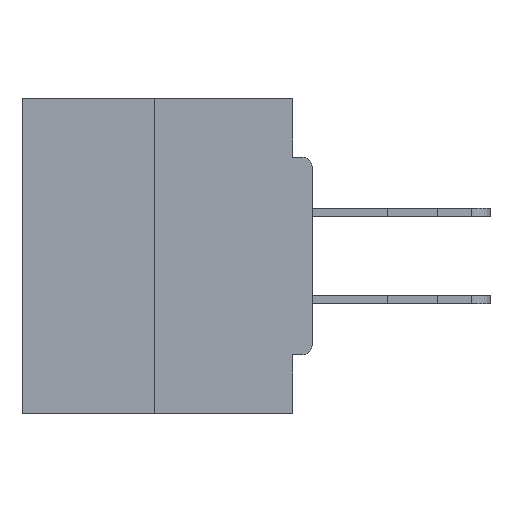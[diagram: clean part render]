
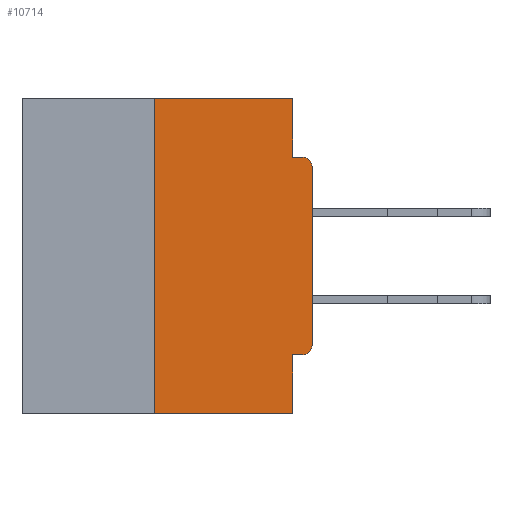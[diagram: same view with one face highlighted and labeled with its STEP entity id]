
A CAD part, left-side view. The second image highlights one B-rep face of the part: STEP entity #10714.
In plain terms, the highlighted planar face has unit normal (-1, 0, 0).
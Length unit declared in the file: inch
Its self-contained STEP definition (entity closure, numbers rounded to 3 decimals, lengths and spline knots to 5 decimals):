
#141 = ORIENTED_EDGE ( 'NONE', *, *, #17769, .T. ) ;
#172 = DIRECTION ( 'NONE',  ( 0., 0., -1. ) ) ;
#173 = DIRECTION ( 'NONE',  ( 0., -1., 0. ) ) ;
#638 = LINE ( 'NONE', #19445, #23452 ) ;
#1188 = CARTESIAN_POINT ( 'NONE',  ( 0., 0., 0. ) ) ;
#2145 = CARTESIAN_POINT ( 'NONE',  ( 0., 0.25, 0. ) ) ;
#2170 = LINE ( 'NONE', #11632, #36227 ) ;
#2729 = DIRECTION ( 'NONE',  ( 0., -1., 0. ) ) ;
#3438 = CARTESIAN_POINT ( 'NONE',  ( 0., 0.015, -0.3915 ) ) ;
#3566 = DIRECTION ( 'NONE',  ( 0., 0., 1. ) ) ;
#4624 = EDGE_CURVE ( 'NONE', #17045, #29672, #16320, .T. ) ;
#4887 = CARTESIAN_POINT ( 'NONE',  ( 0., 0.015, -0.0935 ) ) ;
#5136 = EDGE_CURVE ( 'NONE', #35046, #29506, #31092, .T. ) ;
#5449 = EDGE_CURVE ( 'NONE', #21550, #13218, #638, .T. ) ;
#6110 = AXIS2_PLACEMENT_3D ( 'NONE', #3438, #6583, #9461 ) ;
#6583 = DIRECTION ( 'NONE',  ( -1., 0., 0. ) ) ;
#6952 = CARTESIAN_POINT ( 'NONE',  ( 0., 0.031, -0.5 ) ) ;
#7088 = ORIENTED_EDGE ( 'NONE', *, *, #30338, .T. ) ;
#7801 = DIRECTION ( 'NONE',  ( 0., -1., 0. ) ) ;
#8574 = CIRCLE ( 'NONE', #6110, 0.015 ) ;
#8868 = CARTESIAN_POINT ( 'NONE',  ( 0., 0., -0.4065 ) ) ;
#9128 = CARTESIAN_POINT ( 'NONE',  ( 0., 0.031, -0.4065 ) ) ;
#9140 = EDGE_LOOP ( 'NONE', ( #13196, #24251, #141, #27956, #31343, #7088, #16953, #16206, #29349, #14615 ) ) ;
#9144 = CARTESIAN_POINT ( 'NONE',  ( 0., 0.46, 0. ) ) ;
#9461 = DIRECTION ( 'NONE',  ( 0., 0., -1. ) ) ;
#9578 = CARTESIAN_POINT ( 'NONE',  ( 0., 0.25, -0.5 ) ) ;
#9580 = DIRECTION ( 'NONE',  ( 0., 0., -1. ) ) ;
#9927 = EDGE_CURVE ( 'NONE', #35628, #25838, #33944, .T. ) ;
#10643 = AXIS2_PLACEMENT_3D ( 'NONE', #9144, #23290, #172 ) ;
#10714 = ADVANCED_FACE ( 'NONE', ( #15776 ), #11755, .F. ) ;
#10856 = CARTESIAN_POINT ( 'NONE',  ( 0., 0., -0.3915 ) ) ;
#11632 = CARTESIAN_POINT ( 'NONE',  ( 0., 0.46, -0.5 ) ) ;
#11755 = PLANE ( 'NONE',  #10643 ) ;
#12730 = CARTESIAN_POINT ( 'NONE',  ( 0., 0.031, -0.0935 ) ) ;
#12836 = CARTESIAN_POINT ( 'NONE',  ( 0., 0.46, 0. ) ) ;
#13103 = VERTEX_POINT ( 'NONE', #29888 ) ;
#13196 = ORIENTED_EDGE ( 'NONE', *, *, #21274, .F. ) ;
#13218 = VERTEX_POINT ( 'NONE', #4887 ) ;
#13568 = CIRCLE ( 'NONE', #36245, 0.015 ) ;
#14615 = ORIENTED_EDGE ( 'NONE', *, *, #32724, .F. ) ;
#14978 = DIRECTION ( 'NONE',  ( 0., 0., -1. ) ) ;
#14980 = VECTOR ( 'NONE', #28480, 39.37008 ) ;
#15696 = EDGE_CURVE ( 'NONE', #29672, #34847, #34263, .T. ) ;
#15776 = FACE_OUTER_BOUND ( 'NONE', #9140, .T. ) ;
#16206 = ORIENTED_EDGE ( 'NONE', *, *, #28517, .T. ) ;
#16320 = LINE ( 'NONE', #8868, #14980 ) ;
#16727 = CARTESIAN_POINT ( 'NONE',  ( 0., 0.25, 0. ) ) ;
#16953 = ORIENTED_EDGE ( 'NONE', *, *, #5136, .T. ) ;
#17045 = VERTEX_POINT ( 'NONE', #33713 ) ;
#17710 = VECTOR ( 'NONE', #14978, 39.37008 ) ;
#17769 = EDGE_CURVE ( 'NONE', #35628, #34847, #2170, .T. ) ;
#18042 = DIRECTION ( 'NONE',  ( 0., 0., -1. ) ) ;
#18284 = DIRECTION ( 'NONE',  ( -1., 0., 0. ) ) ;
#19445 = CARTESIAN_POINT ( 'NONE',  ( 0., 0., -0.0935 ) ) ;
#21274 = EDGE_CURVE ( 'NONE', #25838, #13103, #27729, .T. ) ;
#21550 = VERTEX_POINT ( 'NONE', #12730 ) ;
#23290 = DIRECTION ( 'NONE',  ( 1., 0., 0. ) ) ;
#23452 = VECTOR ( 'NONE', #7801, 39.37008 ) ;
#24002 = CARTESIAN_POINT ( 'NONE',  ( 0., 0.031, -0.5 ) ) ;
#24251 = ORIENTED_EDGE ( 'NONE', *, *, #9927, .F. ) ;
#25406 = CARTESIAN_POINT ( 'NONE',  ( 0., 0., -0.1085 ) ) ;
#25838 = VERTEX_POINT ( 'NONE', #16727 ) ;
#26329 = VECTOR ( 'NONE', #30411, 39.37008 ) ;
#26729 = LINE ( 'NONE', #35127, #29843 ) ;
#27729 = LINE ( 'NONE', #12836, #36725 ) ;
#27956 = ORIENTED_EDGE ( 'NONE', *, *, #15696, .F. ) ;
#28369 = VECTOR ( 'NONE', #3566, 39.37008 ) ;
#28480 = DIRECTION ( 'NONE',  ( 0., 1., 0. ) ) ;
#28517 = EDGE_CURVE ( 'NONE', #29506, #13218, #13568, .T. ) ;
#29349 = ORIENTED_EDGE ( 'NONE', *, *, #5449, .F. ) ;
#29506 = VERTEX_POINT ( 'NONE', #25406 ) ;
#29672 = VERTEX_POINT ( 'NONE', #9128 ) ;
#29843 = VECTOR ( 'NONE', #9580, 39.37008 ) ;
#29888 = CARTESIAN_POINT ( 'NONE',  ( 0., 0.031, 0. ) ) ;
#30338 = EDGE_CURVE ( 'NONE', #17045, #35046, #8574, .T. ) ;
#30411 = DIRECTION ( 'NONE',  ( 0., 0., 1. ) ) ;
#31092 = LINE ( 'NONE', #1188, #28369 ) ;
#31343 = ORIENTED_EDGE ( 'NONE', *, *, #4624, .F. ) ;
#32666 = CARTESIAN_POINT ( 'NONE',  ( 0., 0.015, -0.1085 ) ) ;
#32724 = EDGE_CURVE ( 'NONE', #13103, #21550, #26729, .T. ) ;
#33713 = CARTESIAN_POINT ( 'NONE',  ( 0., 0.015, -0.4065 ) ) ;
#33944 = LINE ( 'NONE', #2145, #26329 ) ;
#34263 = LINE ( 'NONE', #24002, #17710 ) ;
#34847 = VERTEX_POINT ( 'NONE', #6952 ) ;
#35046 = VERTEX_POINT ( 'NONE', #10856 ) ;
#35127 = CARTESIAN_POINT ( 'NONE',  ( 0., 0.031, 0. ) ) ;
#35628 = VERTEX_POINT ( 'NONE', #9578 ) ;
#36227 = VECTOR ( 'NONE', #173, 39.37008 ) ;
#36245 = AXIS2_PLACEMENT_3D ( 'NONE', #32666, #18284, #18042 ) ;
#36725 = VECTOR ( 'NONE', #2729, 39.37008 ) ;
